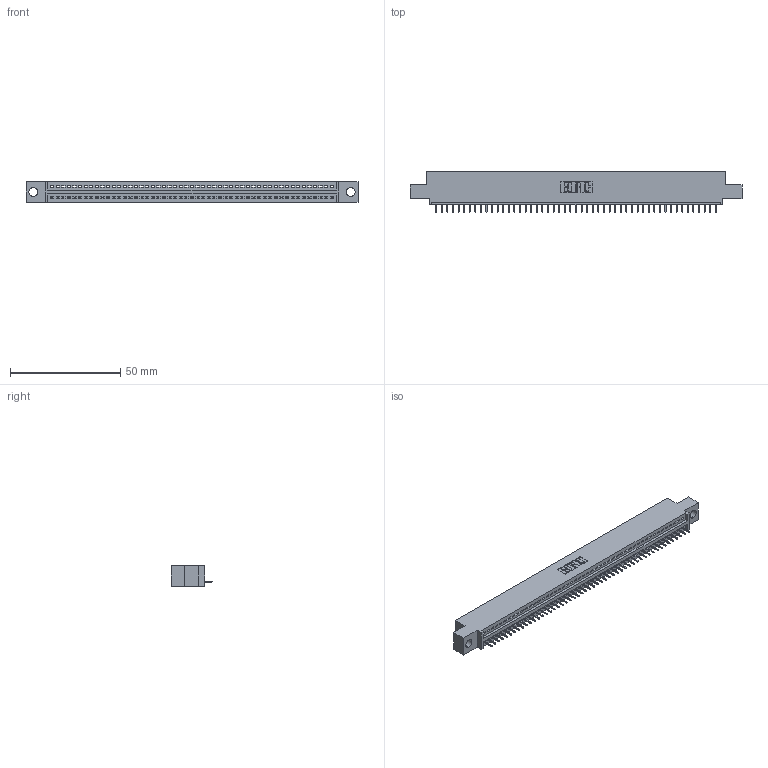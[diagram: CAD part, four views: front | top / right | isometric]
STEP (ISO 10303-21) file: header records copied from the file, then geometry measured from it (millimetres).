
FILE_DESCRIPTION (( 'STEP AP203' ), '1' );
FILE_NAME ('345-051-525-404.STEP', '2020-09-20T03:43:39', ( '' ), ( '' ), 'SwSTEP 2.0', 'SolidWorks 2020', '' );
FILE_SCHEMA (( 'CONFIG_CONTROL_DESIGN' ));
Length unit declared in the file: inch
Products named in the file (3): 345-292-001_345-293-125; 345-051-525-404; 345 Part_0.110 Offset - 0.156 Dia-TH
Assembly tree (52 placements, depth 2):
  345-051-525-404
    345 Part_0.110 Offset - 0.156 Dia-TH
    345-292-001_345-293-125  x51
Bounding box: 150.75 x 18.72 x 9.4 mm (x, y, z)
Volume: 14022.6 mm3; surface area: 17953.3 mm2
Topology: 52 solids, 52 shells, 3292 faces, 9533 edges, 6150 vertices
Faces by surface type: plane 2430, cylinder 862
Entity records: 37381 total; most frequent: CARTESIAN_POINT 6481, ORIENTED_EDGE 6466, DIRECTION 5647, EDGE_CURVE 3233, LINE 2901, VECTOR 2901, VERTEX_POINT 2150, AXIS2_PLACEMENT_3D 1373
